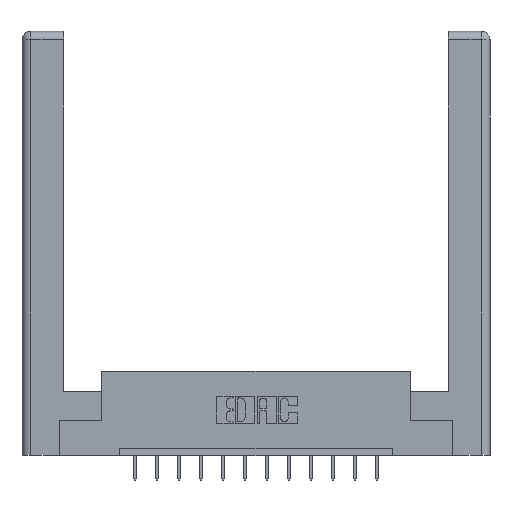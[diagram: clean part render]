
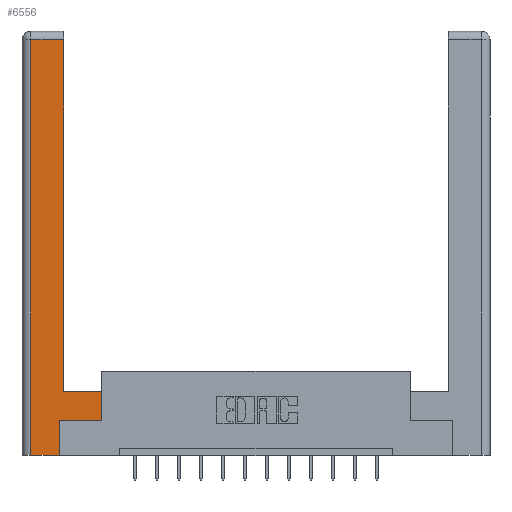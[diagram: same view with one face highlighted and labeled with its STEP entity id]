
A CAD part, top view. The second image highlights one B-rep face of the part: STEP entity #6556.
In plain terms, the highlighted planar face has unit normal (0, 0, 1).
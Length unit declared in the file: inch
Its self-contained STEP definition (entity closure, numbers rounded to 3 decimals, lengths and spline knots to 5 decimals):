
#73 = DIRECTION ( 'NONE',  ( 1., 0., 0. ) ) ;
#258 = EDGE_LOOP ( 'NONE', ( #558, #10372, #9797, #4587, #5412, #593, #2418, #3178 ) ) ;
#277 = VERTEX_POINT ( 'NONE', #7763 ) ;
#280 = LINE ( 'NONE', #3606, #12641 ) ;
#405 = VERTEX_POINT ( 'NONE', #3674 ) ;
#558 = ORIENTED_EDGE ( 'NONE', *, *, #9598, .T. ) ;
#593 = ORIENTED_EDGE ( 'NONE', *, *, #898, .T. ) ;
#898 = EDGE_CURVE ( 'NONE', #8659, #6350, #280, .T. ) ;
#951 = VECTOR ( 'NONE', #2335, 39.37008 ) ;
#1324 = LINE ( 'NONE', #10358, #13313 ) ;
#1776 = DIRECTION ( 'NONE',  ( 0., -1., 0. ) ) ;
#1778 = VERTEX_POINT ( 'NONE', #6324 ) ;
#1958 = VECTOR ( 'NONE', #5588, 39.37008 ) ;
#2335 = DIRECTION ( 'NONE',  ( 0., 1., 0. ) ) ;
#2418 = ORIENTED_EDGE ( 'NONE', *, *, #8304, .T. ) ;
#2836 = LINE ( 'NONE', #4301, #7325 ) ;
#2985 = CARTESIAN_POINT ( 'NONE',  ( 0.265, 0., 0. ) ) ;
#3132 = VERTEX_POINT ( 'NONE', #8111 ) ;
#3178 = ORIENTED_EDGE ( 'NONE', *, *, #7015, .T. ) ;
#3324 = VERTEX_POINT ( 'NONE', #3678 ) ;
#3592 = DIRECTION ( 'NONE',  ( -1., 0., 0. ) ) ;
#3606 = CARTESIAN_POINT ( 'NONE',  ( 0.565, 0.245, 0. ) ) ;
#3673 = EDGE_CURVE ( 'NONE', #277, #1778, #2836, .T. ) ;
#3674 = CARTESIAN_POINT ( 'NONE',  ( 0.265, 0., 0. ) ) ;
#3678 = CARTESIAN_POINT ( 'NONE',  ( 0.295, 0.45, 0. ) ) ;
#4025 = LINE ( 'NONE', #2985, #6827 ) ;
#4301 = CARTESIAN_POINT ( 'NONE',  ( 0.0615, 0., 0. ) ) ;
#4429 = CARTESIAN_POINT ( 'NONE',  ( 0.265, 0.245, 0. ) ) ;
#4587 = ORIENTED_EDGE ( 'NONE', *, *, #12823, .T. ) ;
#4717 = CARTESIAN_POINT ( 'NONE',  ( 0.295, 3., 0. ) ) ;
#5185 = VERTEX_POINT ( 'NONE', #13033 ) ;
#5412 = ORIENTED_EDGE ( 'NONE', *, *, #11629, .T. ) ;
#5588 = DIRECTION ( 'NONE',  ( -1., 0., 0. ) ) ;
#5981 = LINE ( 'NONE', #8183, #8216 ) ;
#6274 = LINE ( 'NONE', #13958, #1958 ) ;
#6324 = CARTESIAN_POINT ( 'NONE',  ( 0.0615, 0., 0. ) ) ;
#6350 = VERTEX_POINT ( 'NONE', #7275 ) ;
#6556 = ADVANCED_FACE ( 'NONE', ( #10579 ), #13298, .F. ) ;
#6827 = VECTOR ( 'NONE', #7533, 39.37008 ) ;
#7015 = EDGE_CURVE ( 'NONE', #5185, #3324, #6274, .T. ) ;
#7275 = CARTESIAN_POINT ( 'NONE',  ( 0.565, 0.245, 0. ) ) ;
#7325 = VECTOR ( 'NONE', #1776, 39.37008 ) ;
#7533 = DIRECTION ( 'NONE',  ( 1., 0., 0. ) ) ;
#7763 = CARTESIAN_POINT ( 'NONE',  ( 0.0615, 2.94, 0. ) ) ;
#8111 = CARTESIAN_POINT ( 'NONE',  ( 0.295, 2.94, 0. ) ) ;
#8183 = CARTESIAN_POINT ( 'NONE',  ( 0.0615, 2.94, 0. ) ) ;
#8216 = VECTOR ( 'NONE', #15297, 39.37008 ) ;
#8304 = EDGE_CURVE ( 'NONE', #6350, #5185, #1324, .T. ) ;
#8343 = CARTESIAN_POINT ( 'NONE',  ( 0., 0., 0. ) ) ;
#8387 = AXIS2_PLACEMENT_3D ( 'NONE', #8343, #9745, #3592 ) ;
#8659 = VERTEX_POINT ( 'NONE', #4429 ) ;
#8740 = VECTOR ( 'NONE', #14450, 39.37008 ) ;
#9598 = EDGE_CURVE ( 'NONE', #3324, #3132, #13855, .T. ) ;
#9745 = DIRECTION ( 'NONE',  ( 0., 0., -1. ) ) ;
#9797 = ORIENTED_EDGE ( 'NONE', *, *, #3673, .T. ) ;
#9850 = LINE ( 'NONE', #14294, #8740 ) ;
#9860 = EDGE_CURVE ( 'NONE', #3132, #277, #5981, .T. ) ;
#10358 = CARTESIAN_POINT ( 'NONE',  ( 0.565, 0.45, 0. ) ) ;
#10372 = ORIENTED_EDGE ( 'NONE', *, *, #9860, .T. ) ;
#10579 = FACE_OUTER_BOUND ( 'NONE', #258, .T. ) ;
#11629 = EDGE_CURVE ( 'NONE', #405, #8659, #9850, .T. ) ;
#12641 = VECTOR ( 'NONE', #73, 39.37008 ) ;
#12806 = DIRECTION ( 'NONE',  ( 0., 1., 0. ) ) ;
#12823 = EDGE_CURVE ( 'NONE', #1778, #405, #4025, .T. ) ;
#13033 = CARTESIAN_POINT ( 'NONE',  ( 0.565, 0.45, 0. ) ) ;
#13298 = PLANE ( 'NONE',  #8387 ) ;
#13313 = VECTOR ( 'NONE', #12806, 39.37008 ) ;
#13855 = LINE ( 'NONE', #4717, #951 ) ;
#13958 = CARTESIAN_POINT ( 'NONE',  ( 0.295, 0.45, 0. ) ) ;
#14294 = CARTESIAN_POINT ( 'NONE',  ( 0.265, 0.245, 0. ) ) ;
#14450 = DIRECTION ( 'NONE',  ( 0., 1., 0. ) ) ;
#15297 = DIRECTION ( 'NONE',  ( -1., 0., 0. ) ) ;
